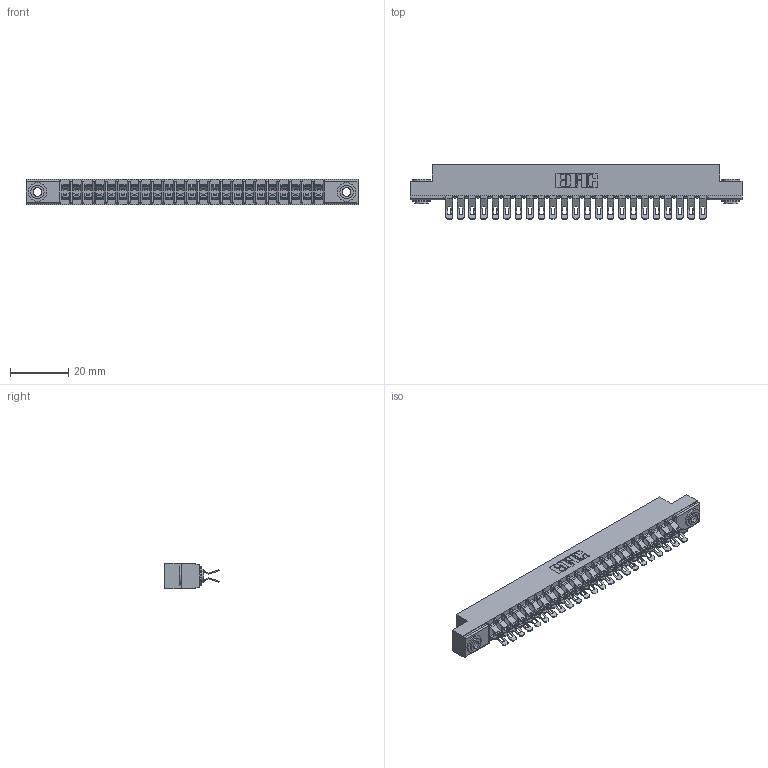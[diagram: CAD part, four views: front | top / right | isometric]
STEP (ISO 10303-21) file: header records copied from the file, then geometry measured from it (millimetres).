
FILE_DESCRIPTION (( 'STEP AP203' ), '1' );
FILE_NAME ('307-046-455-203.STEP', '2020-09-30T02:33:32', ( '' ), ( '' ), 'SwSTEP 2.0', 'SolidWorks 2020', '' );
FILE_SCHEMA (( 'CONFIG_CONTROL_DESIGN' ));
Length unit declared in the file: inch
Products named in the file (4): 307 Part_.156 Dia Mounting Holes; 307-046-455-203; 307-290-001_555; 345-250-002_345-250-002-102
Assembly tree (49 placements, depth 2):
  307-046-455-203
    307 Part_.156 Dia Mounting Holes
    307-290-001_555  x46
    345-250-002_345-250-002-102  x2
Bounding box: 114.15 x 18.75 x 8.71 mm (x, y, z)
Volume: 7604.7 mm3; surface area: 14488.2 mm2
Topology: 49 solids, 49 shells, 3000 faces, 8761 edges, 5710 vertices
Faces by surface type: plane 1658, cylinder 1286, sphere 48, cone 8
Entity records: 24398 total; most frequent: CARTESIAN_POINT 3984, ORIENTED_EDGE 3940, DIRECTION 3932, EDGE_CURVE 1970, VECTOR 1484, LINE 1484, VERTEX_POINT 1276, AXIS2_PLACEMENT_3D 1224
